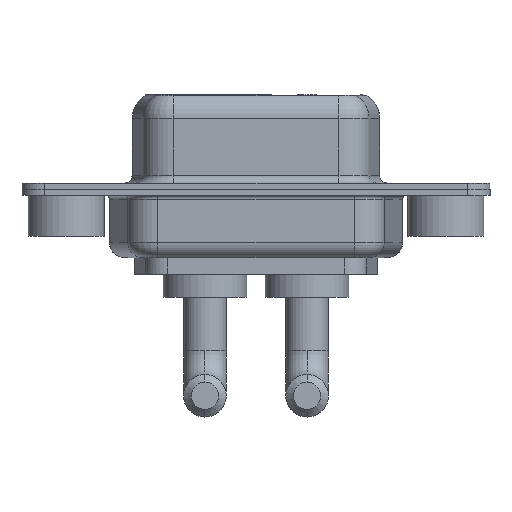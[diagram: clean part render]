
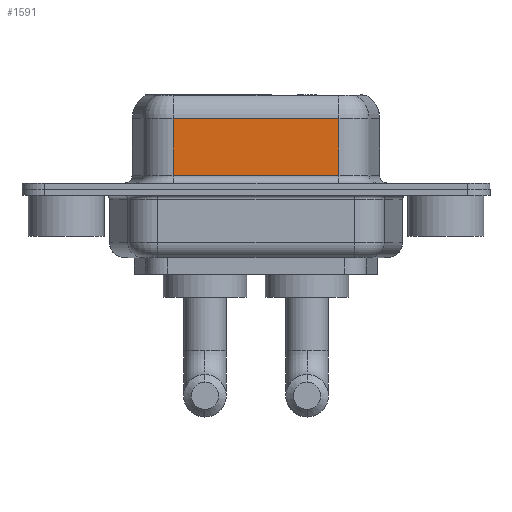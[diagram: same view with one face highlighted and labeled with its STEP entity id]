
A CAD part, front view. The second image highlights one B-rep face of the part: STEP entity #1591.
In plain terms, the highlighted planar face has unit normal (0, -1, 0).
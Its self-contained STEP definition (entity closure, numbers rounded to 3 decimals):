
#956 = VECTOR ( 'NONE', #4771, 1000. ) ;
#1441 = CARTESIAN_POINT ( 'NONE',  ( 7.038, -3.95, 0.9 ) ) ;
#1591 = ADVANCED_FACE ( 'NONE', ( #6268 ), #10354, .F. ) ;
#1687 = CARTESIAN_POINT ( 'NONE',  ( 17.962, -3.95, 4.65 ) ) ;
#2077 = VECTOR ( 'NONE', #3365, 1000. ) ;
#2191 = CARTESIAN_POINT ( 'NONE',  ( 17.962, -3.95, 0.9 ) ) ;
#2832 = AXIS2_PLACEMENT_3D ( 'NONE', #9204, #12250, #9408 ) ;
#3365 = DIRECTION ( 'NONE',  ( -1., 0., 0. ) ) ;
#3545 = VERTEX_POINT ( 'NONE', #1687 ) ;
#3689 = CARTESIAN_POINT ( 'NONE',  ( 7.038, -3.95, 6.4 ) ) ;
#3897 = ORIENTED_EDGE ( 'NONE', *, *, #4545, .F. ) ;
#4183 = VECTOR ( 'NONE', #8625, 1000. ) ;
#4244 = ORIENTED_EDGE ( 'NONE', *, *, #7030, .T. ) ;
#4456 = CARTESIAN_POINT ( 'NONE',  ( 7.038, -3.95, 4.65 ) ) ;
#4545 = EDGE_CURVE ( 'NONE', #3545, #10766, #9160, .T. ) ;
#4711 = LINE ( 'NONE', #3689, #956 ) ;
#4756 = VERTEX_POINT ( 'NONE', #1441 ) ;
#4771 = DIRECTION ( 'NONE',  ( 0., 0., -1. ) ) ;
#5632 = CARTESIAN_POINT ( 'NONE',  ( 17.962, -3.95, 0.9 ) ) ;
#5648 = EDGE_CURVE ( 'NONE', #4756, #10766, #12824, .T. ) ;
#6268 = FACE_OUTER_BOUND ( 'NONE', #12076, .T. ) ;
#6647 = CARTESIAN_POINT ( 'NONE',  ( 17.962, -3.95, 4.65 ) ) ;
#7030 = EDGE_CURVE ( 'NONE', #3545, #9553, #10680, .T. ) ;
#8414 = CARTESIAN_POINT ( 'NONE',  ( 17.962, -3.95, 6.4 ) ) ;
#8625 = DIRECTION ( 'NONE',  ( 1., 0., 0. ) ) ;
#9160 = LINE ( 'NONE', #8414, #12760 ) ;
#9204 = CARTESIAN_POINT ( 'NONE',  ( 17.962, -3.95, 6.4 ) ) ;
#9408 = DIRECTION ( 'NONE',  ( -1., 0., 0. ) ) ;
#9553 = VERTEX_POINT ( 'NONE', #4456 ) ;
#10354 = PLANE ( 'NONE',  #2832 ) ;
#10680 = LINE ( 'NONE', #6647, #2077 ) ;
#10766 = VERTEX_POINT ( 'NONE', #2191 ) ;
#11459 = DIRECTION ( 'NONE',  ( 0., 0., -1. ) ) ;
#11737 = ORIENTED_EDGE ( 'NONE', *, *, #5648, .T. ) ;
#12076 = EDGE_LOOP ( 'NONE', ( #3897, #4244, #12533, #11737 ) ) ;
#12250 = DIRECTION ( 'NONE',  ( 0., 1., 0. ) ) ;
#12303 = EDGE_CURVE ( 'NONE', #9553, #4756, #4711, .T. ) ;
#12533 = ORIENTED_EDGE ( 'NONE', *, *, #12303, .T. ) ;
#12760 = VECTOR ( 'NONE', #11459, 1000. ) ;
#12824 = LINE ( 'NONE', #5632, #4183 ) ;
